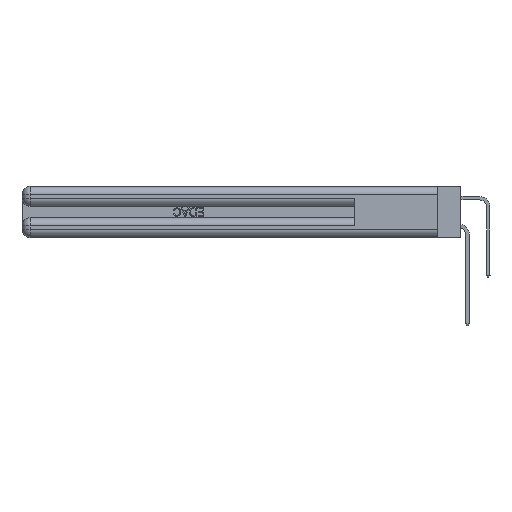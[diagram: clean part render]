
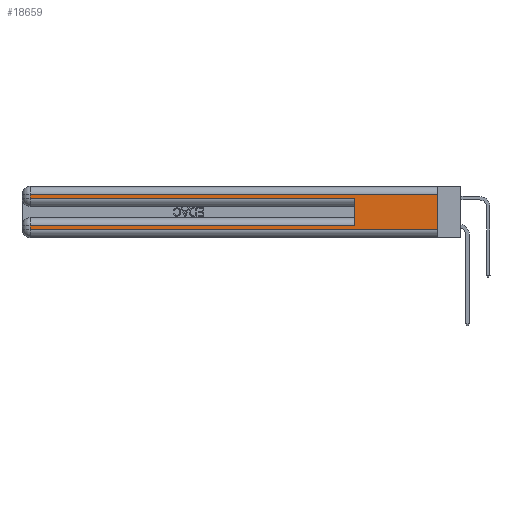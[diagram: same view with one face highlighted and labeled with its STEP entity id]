
A CAD part, left-side view. The second image highlights one B-rep face of the part: STEP entity #18659.
In plain terms, the highlighted planar face has unit normal (-1, 0, 0).
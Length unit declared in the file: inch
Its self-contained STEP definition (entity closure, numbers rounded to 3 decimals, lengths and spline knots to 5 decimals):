
#72 = EDGE_CURVE ( 'NONE', #7595, #8122, #38800, .T. ) ;
#342 = EDGE_CURVE ( 'NONE', #3057, #5038, #21444, .T. ) ;
#1783 = ORIENTED_EDGE ( 'NONE', *, *, #12855, .T. ) ;
#2824 = CARTESIAN_POINT ( 'NONE',  ( 0., 0.6, 0.285 ) ) ;
#3057 = VERTEX_POINT ( 'NONE', #39462 ) ;
#4014 = ORIENTED_EDGE ( 'NONE', *, *, #21924, .F. ) ;
#4473 = DIRECTION ( 'NONE',  ( 0., -1., 0. ) ) ;
#4722 = LINE ( 'NONE', #27297, #27894 ) ;
#4743 = CARTESIAN_POINT ( 'NONE',  ( 0., 0., 0.31 ) ) ;
#4800 = CARTESIAN_POINT ( 'NONE',  ( 0., 2.94, 0.37 ) ) ;
#5038 = VERTEX_POINT ( 'NONE', #22933 ) ;
#6963 = DIRECTION ( 'NONE',  ( 0., -1., 0. ) ) ;
#7595 = VERTEX_POINT ( 'NONE', #17180 ) ;
#8122 = VERTEX_POINT ( 'NONE', #35925 ) ;
#10006 = CARTESIAN_POINT ( 'NONE',  ( 0., 2.94, 0.285 ) ) ;
#10567 = EDGE_CURVE ( 'NONE', #3057, #21362, #16226, .T. ) ;
#11259 = VECTOR ( 'NONE', #31658, 39.37008 ) ;
#12855 = EDGE_CURVE ( 'NONE', #31113, #18888, #32457, .T. ) ;
#14090 = ORIENTED_EDGE ( 'NONE', *, *, #342, .F. ) ;
#14877 = VECTOR ( 'NONE', #6963, 39.37008 ) ;
#15034 = DIRECTION ( 'NONE',  ( 0., 0., 1. ) ) ;
#15105 = DIRECTION ( 'NONE',  ( 1., 0., 0. ) ) ;
#15274 = CARTESIAN_POINT ( 'NONE',  ( 0., 0., 0.085 ) ) ;
#16226 = LINE ( 'NONE', #4743, #26404 ) ;
#16414 = EDGE_CURVE ( 'NONE', #21362, #31113, #25474, .T. ) ;
#16581 = DIRECTION ( 'NONE',  ( 0., 1., 0. ) ) ;
#17098 = CARTESIAN_POINT ( 'NONE',  ( 0., 2.94, 0.31 ) ) ;
#17180 = CARTESIAN_POINT ( 'NONE',  ( 0., 2.94, 0.085 ) ) ;
#17770 = VECTOR ( 'NONE', #21912, 39.37008 ) ;
#17800 = CARTESIAN_POINT ( 'NONE',  ( 0., 2.94, 0.37 ) ) ;
#17806 = VECTOR ( 'NONE', #28045, 39.37008 ) ;
#18659 = ADVANCED_FACE ( 'NONE', ( #32941 ), #34021, .F. ) ;
#18752 = ORIENTED_EDGE ( 'NONE', *, *, #10567, .T. ) ;
#18888 = VERTEX_POINT ( 'NONE', #2824 ) ;
#20147 = CARTESIAN_POINT ( 'NONE',  ( 0., 0.6, 0.085 ) ) ;
#20481 = ORIENTED_EDGE ( 'NONE', *, *, #30852, .T. ) ;
#20895 = DIRECTION ( 'NONE',  ( 0., 0., -1. ) ) ;
#21131 = ORIENTED_EDGE ( 'NONE', *, *, #16414, .T. ) ;
#21362 = VERTEX_POINT ( 'NONE', #17098 ) ;
#21444 = LINE ( 'NONE', #35918, #11259 ) ;
#21912 = DIRECTION ( 'NONE',  ( 0., 0., -1. ) ) ;
#21924 = EDGE_CURVE ( 'NONE', #34430, #18888, #4722, .T. ) ;
#22668 = EDGE_LOOP ( 'NONE', ( #14090, #18752, #21131, #1783, #4014, #20481, #29735, #35760 ) ) ;
#22903 = EDGE_CURVE ( 'NONE', #8122, #5038, #37491, .T. ) ;
#22933 = CARTESIAN_POINT ( 'NONE',  ( 0., 0., 0.06 ) ) ;
#24326 = VECTOR ( 'NONE', #4473, 39.37008 ) ;
#24601 = CARTESIAN_POINT ( 'NONE',  ( 0., 0., 0.06 ) ) ;
#25474 = LINE ( 'NONE', #4800, #17770 ) ;
#26404 = VECTOR ( 'NONE', #16581, 39.37008 ) ;
#26953 = AXIS2_PLACEMENT_3D ( 'NONE', #33516, #15105, #36651 ) ;
#27297 = CARTESIAN_POINT ( 'NONE',  ( 0., 0.6, 0.145 ) ) ;
#27894 = VECTOR ( 'NONE', #15034, 39.37008 ) ;
#28045 = DIRECTION ( 'NONE',  ( 0., 1., 0. ) ) ;
#29735 = ORIENTED_EDGE ( 'NONE', *, *, #72, .T. ) ;
#30604 = VECTOR ( 'NONE', #20895, 39.37008 ) ;
#30852 = EDGE_CURVE ( 'NONE', #34430, #7595, #38526, .T. ) ;
#31113 = VERTEX_POINT ( 'NONE', #10006 ) ;
#31658 = DIRECTION ( 'NONE',  ( 0., 0., -1. ) ) ;
#32457 = LINE ( 'NONE', #34510, #24326 ) ;
#32941 = FACE_OUTER_BOUND ( 'NONE', #22668, .T. ) ;
#33516 = CARTESIAN_POINT ( 'NONE',  ( 0., 0., 0.37 ) ) ;
#34021 = PLANE ( 'NONE',  #26953 ) ;
#34430 = VERTEX_POINT ( 'NONE', #20147 ) ;
#34510 = CARTESIAN_POINT ( 'NONE',  ( 0., 0., 0.285 ) ) ;
#35760 = ORIENTED_EDGE ( 'NONE', *, *, #22903, .T. ) ;
#35918 = CARTESIAN_POINT ( 'NONE',  ( 0., 0., 0.37 ) ) ;
#35925 = CARTESIAN_POINT ( 'NONE',  ( 0., 2.94, 0.06 ) ) ;
#36651 = DIRECTION ( 'NONE',  ( 0., 0., -1. ) ) ;
#37491 = LINE ( 'NONE', #24601, #14877 ) ;
#38526 = LINE ( 'NONE', #15274, #17806 ) ;
#38800 = LINE ( 'NONE', #17800, #30604 ) ;
#39462 = CARTESIAN_POINT ( 'NONE',  ( 0., 0., 0.31 ) ) ;
